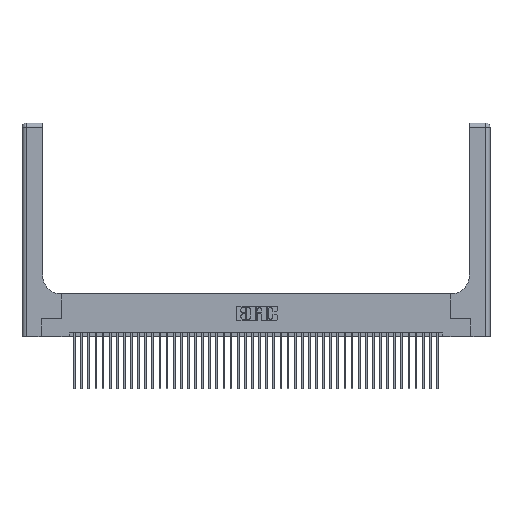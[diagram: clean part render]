
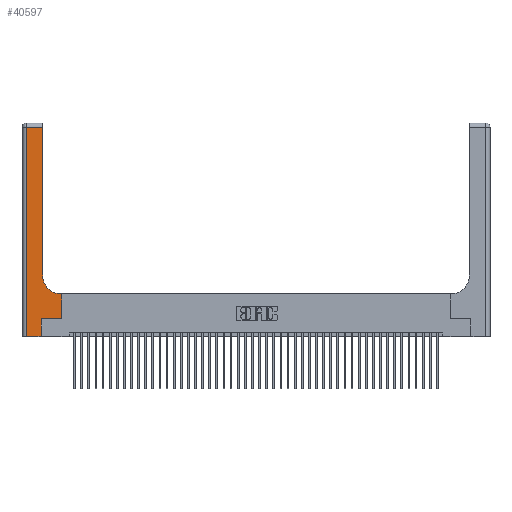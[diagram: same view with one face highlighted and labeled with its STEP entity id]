
A CAD part, top view. The second image highlights one B-rep face of the part: STEP entity #40597.
In plain terms, the highlighted planar face has unit normal (0, 0, 1).
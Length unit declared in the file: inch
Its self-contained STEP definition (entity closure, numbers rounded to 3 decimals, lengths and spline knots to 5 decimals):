
#237 = VERTEX_POINT ( 'NONE', #38672 ) ;
#721 = LINE ( 'NONE', #22284, #16437 ) ;
#879 = CIRCLE ( 'NONE', #14967, 0.25 ) ;
#934 = EDGE_CURVE ( 'NONE', #237, #36676, #879, .T. ) ;
#1595 = LINE ( 'NONE', #6881, #42047 ) ;
#2098 = CARTESIAN_POINT ( 'NONE',  ( 0.5415, 0.85, 0.37 ) ) ;
#2353 = VECTOR ( 'NONE', #28835, 39.37008 ) ;
#3212 = VERTEX_POINT ( 'NONE', #37743 ) ;
#3584 = DIRECTION ( 'NONE',  ( 0., 1., 0. ) ) ;
#3627 = LINE ( 'NONE', #21251, #7392 ) ;
#4726 = EDGE_CURVE ( 'NONE', #16063, #9958, #29237, .T. ) ;
#5580 = DIRECTION ( 'NONE',  ( 1., 0., 0. ) ) ;
#6231 = ORIENTED_EDGE ( 'NONE', *, *, #19852, .T. ) ;
#6881 = CARTESIAN_POINT ( 'NONE',  ( 0.5585, 0.25, 0.37 ) ) ;
#7371 = ORIENTED_EDGE ( 'NONE', *, *, #39734, .T. ) ;
#7392 = VECTOR ( 'NONE', #25008, 39.37008 ) ;
#8718 = DIRECTION ( 'NONE',  ( 0., 0., -1. ) ) ;
#9345 = CARTESIAN_POINT ( 'NONE',  ( 0.269, 0., 0.37 ) ) ;
#9958 = VERTEX_POINT ( 'NONE', #19246 ) ;
#10560 = ORIENTED_EDGE ( 'NONE', *, *, #37190, .T. ) ;
#11456 = VERTEX_POINT ( 'NONE', #15864 ) ;
#12436 = VECTOR ( 'NONE', #44628, 39.37008 ) ;
#12863 = CARTESIAN_POINT ( 'NONE',  ( 0.2915, 0.85, 0.37 ) ) ;
#14853 = CARTESIAN_POINT ( 'NONE',  ( 0., 3., 0.37 ) ) ;
#14967 = AXIS2_PLACEMENT_3D ( 'NONE', #2098, #8718, #5580 ) ;
#15592 = CARTESIAN_POINT ( 'NONE',  ( 0.2915, 0.6, 0.37 ) ) ;
#15749 = VECTOR ( 'NONE', #18465, 39.37008 ) ;
#15864 = CARTESIAN_POINT ( 'NONE',  ( 0.269, 0., 0.37 ) ) ;
#16063 = VERTEX_POINT ( 'NONE', #32413 ) ;
#16437 = VECTOR ( 'NONE', #22872, 39.37008 ) ;
#17104 = EDGE_CURVE ( 'NONE', #43510, #3212, #1595, .T. ) ;
#17340 = CARTESIAN_POINT ( 'NONE',  ( 0.06, 0., 0.37 ) ) ;
#17538 = LINE ( 'NONE', #39849, #43989 ) ;
#18354 = DIRECTION ( 'NONE',  ( 0., 0., -1. ) ) ;
#18465 = DIRECTION ( 'NONE',  ( -1., 0., 0. ) ) ;
#19246 = CARTESIAN_POINT ( 'NONE',  ( 0.06, 2.94, 0.37 ) ) ;
#19771 = DIRECTION ( 'NONE',  ( 0., 1., 0. ) ) ;
#19852 = EDGE_CURVE ( 'NONE', #3212, #237, #21779, .T. ) ;
#20876 = ORIENTED_EDGE ( 'NONE', *, *, #4726, .T. ) ;
#21251 = CARTESIAN_POINT ( 'NONE',  ( 0.269, 0.25, 0.37 ) ) ;
#21679 = EDGE_LOOP ( 'NONE', ( #39018, #20876, #25954, #7371, #25547, #10560, #39070, #6231, #25611 ) ) ;
#21779 = LINE ( 'NONE', #15592, #2353 ) ;
#22284 = CARTESIAN_POINT ( 'NONE',  ( 0., 0., 0.37 ) ) ;
#22872 = DIRECTION ( 'NONE',  ( 1., 0., 0. ) ) ;
#25008 = DIRECTION ( 'NONE',  ( 1., 0., 0. ) ) ;
#25125 = PLANE ( 'NONE',  #43310 ) ;
#25547 = ORIENTED_EDGE ( 'NONE', *, *, #42038, .T. ) ;
#25611 = ORIENTED_EDGE ( 'NONE', *, *, #934, .T. ) ;
#25954 = ORIENTED_EDGE ( 'NONE', *, *, #26622, .T. ) ;
#26622 = EDGE_CURVE ( 'NONE', #9958, #33917, #38897, .T. ) ;
#26738 = DIRECTION ( 'NONE',  ( 0., -1., 0. ) ) ;
#28139 = FACE_OUTER_BOUND ( 'NONE', #21679, .T. ) ;
#28835 = DIRECTION ( 'NONE',  ( -1., 0., 0. ) ) ;
#29020 = CARTESIAN_POINT ( 'NONE',  ( 0.5585, 0.25, 0.37 ) ) ;
#29237 = LINE ( 'NONE', #29459, #15749 ) ;
#29459 = CARTESIAN_POINT ( 'NONE',  ( 0., 2.94, 0.37 ) ) ;
#30197 = EDGE_CURVE ( 'NONE', #36676, #16063, #17538, .T. ) ;
#31324 = LINE ( 'NONE', #9345, #12436 ) ;
#32413 = CARTESIAN_POINT ( 'NONE',  ( 0.2915, 2.94, 0.37 ) ) ;
#33917 = VERTEX_POINT ( 'NONE', #17340 ) ;
#34939 = CARTESIAN_POINT ( 'NONE',  ( 0.269, 0.25, 0.37 ) ) ;
#36676 = VERTEX_POINT ( 'NONE', #12863 ) ;
#37190 = EDGE_CURVE ( 'NONE', #42220, #43510, #3627, .T. ) ;
#37743 = CARTESIAN_POINT ( 'NONE',  ( 0.5585, 0.6, 0.37 ) ) ;
#37837 = VECTOR ( 'NONE', #26738, 39.37008 ) ;
#38672 = CARTESIAN_POINT ( 'NONE',  ( 0.5415, 0.6, 0.37 ) ) ;
#38897 = LINE ( 'NONE', #43790, #37837 ) ;
#39018 = ORIENTED_EDGE ( 'NONE', *, *, #30197, .T. ) ;
#39070 = ORIENTED_EDGE ( 'NONE', *, *, #17104, .T. ) ;
#39734 = EDGE_CURVE ( 'NONE', #33917, #11456, #721, .T. ) ;
#39849 = CARTESIAN_POINT ( 'NONE',  ( 0.2915, 3., 0.37 ) ) ;
#40597 = ADVANCED_FACE ( 'NONE', ( #28139 ), #25125, .F. ) ;
#42038 = EDGE_CURVE ( 'NONE', #11456, #42220, #31324, .T. ) ;
#42047 = VECTOR ( 'NONE', #3584, 39.37008 ) ;
#42220 = VERTEX_POINT ( 'NONE', #34939 ) ;
#42485 = DIRECTION ( 'NONE',  ( -1., 0., 0. ) ) ;
#43310 = AXIS2_PLACEMENT_3D ( 'NONE', #14853, #18354, #42485 ) ;
#43510 = VERTEX_POINT ( 'NONE', #29020 ) ;
#43790 = CARTESIAN_POINT ( 'NONE',  ( 0.06, 3., 0.37 ) ) ;
#43989 = VECTOR ( 'NONE', #19771, 39.37008 ) ;
#44628 = DIRECTION ( 'NONE',  ( 0., 1., 0. ) ) ;
